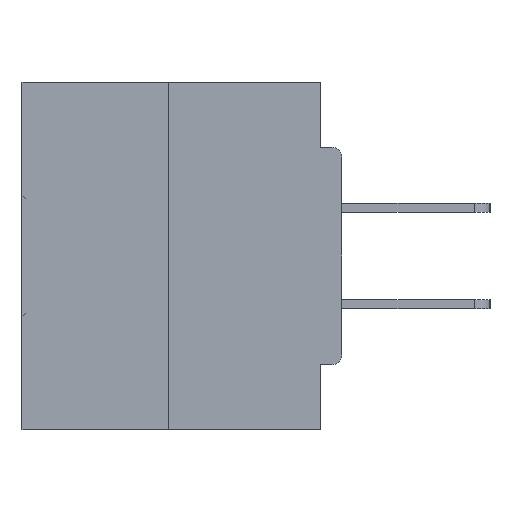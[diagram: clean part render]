
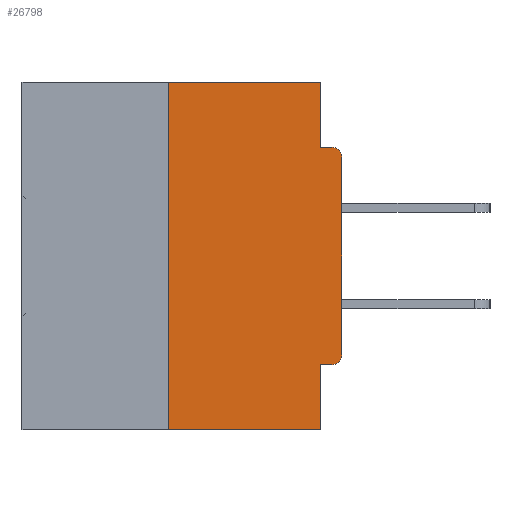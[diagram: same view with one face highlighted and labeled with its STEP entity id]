
A CAD part, left-side view. The second image highlights one B-rep face of the part: STEP entity #26798.
In plain terms, the highlighted planar face has unit normal (-1, 0, 0).
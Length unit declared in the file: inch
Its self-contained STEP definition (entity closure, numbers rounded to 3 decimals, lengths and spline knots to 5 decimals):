
#887 = LINE ( 'NONE', #7431, #6098 ) ;
#1137 = VERTEX_POINT ( 'NONE', #24487 ) ;
#1138 = ORIENTED_EDGE ( 'NONE', *, *, #22868, .F. ) ;
#1396 = DIRECTION ( 'NONE',  ( 0., 0., -1. ) ) ;
#2634 = AXIS2_PLACEMENT_3D ( 'NONE', #39475, #12281, #22226 ) ;
#2792 = ORIENTED_EDGE ( 'NONE', *, *, #13801, .T. ) ;
#3050 = ORIENTED_EDGE ( 'NONE', *, *, #20213, .F. ) ;
#3106 = CARTESIAN_POINT ( 'NONE',  ( 0., 0., -0.4065 ) ) ;
#3130 = VERTEX_POINT ( 'NONE', #12246 ) ;
#3307 = VERTEX_POINT ( 'NONE', #12253 ) ;
#3543 = EDGE_CURVE ( 'NONE', #22917, #3307, #18586, .T. ) ;
#3887 = AXIS2_PLACEMENT_3D ( 'NONE', #36619, #22894, #29551 ) ;
#4044 = VERTEX_POINT ( 'NONE', #23950 ) ;
#4377 = VERTEX_POINT ( 'NONE', #38327 ) ;
#4895 = VERTEX_POINT ( 'NONE', #5065 ) ;
#5065 = CARTESIAN_POINT ( 'NONE',  ( 0., 0., -0.3915 ) ) ;
#5417 = DIRECTION ( 'NONE',  ( 1., 0., 0. ) ) ;
#6098 = VECTOR ( 'NONE', #27663, 39.37008 ) ;
#7431 = CARTESIAN_POINT ( 'NONE',  ( 0., 0.031, 0. ) ) ;
#7897 = CARTESIAN_POINT ( 'NONE',  ( 0., 0.031, -0.5 ) ) ;
#8115 = VECTOR ( 'NONE', #10540, 39.37008 ) ;
#9086 = VERTEX_POINT ( 'NONE', #32831 ) ;
#9930 = DIRECTION ( 'NONE',  ( 0., 1., 0. ) ) ;
#9989 = EDGE_CURVE ( 'NONE', #4895, #4377, #43073, .T. ) ;
#10431 = CARTESIAN_POINT ( 'NONE',  ( 0., 0.25, 0. ) ) ;
#10540 = DIRECTION ( 'NONE',  ( 0., 0., 1. ) ) ;
#10951 = LINE ( 'NONE', #12282, #24762 ) ;
#12246 = CARTESIAN_POINT ( 'NONE',  ( 0., 0.015, -0.0935 ) ) ;
#12253 = CARTESIAN_POINT ( 'NONE',  ( 0., 0.031, -0.4065 ) ) ;
#12281 = DIRECTION ( 'NONE',  ( -1., 0., 0. ) ) ;
#12282 = CARTESIAN_POINT ( 'NONE',  ( 0., 0.46, -0.5 ) ) ;
#13551 = CARTESIAN_POINT ( 'NONE',  ( 0., 0., -0.0935 ) ) ;
#13801 = EDGE_CURVE ( 'NONE', #4044, #25861, #10951, .T. ) ;
#14295 = CARTESIAN_POINT ( 'NONE',  ( 0., 0., 0. ) ) ;
#14833 = FACE_OUTER_BOUND ( 'NONE', #15246, .T. ) ;
#15246 = EDGE_LOOP ( 'NONE', ( #38923, #3050, #2792, #34769, #36209, #39781, #43859, #40238, #1138, #22539 ) ) ;
#15605 = LINE ( 'NONE', #26620, #20967 ) ;
#17031 = EDGE_CURVE ( 'NONE', #3307, #25861, #29061, .T. ) ;
#17248 = LINE ( 'NONE', #13551, #43148 ) ;
#18035 = EDGE_CURVE ( 'NONE', #22917, #4895, #23677, .T. ) ;
#18586 = LINE ( 'NONE', #3106, #29183 ) ;
#20213 = EDGE_CURVE ( 'NONE', #4044, #42009, #39840, .T. ) ;
#20967 = VECTOR ( 'NONE', #30167, 39.37008 ) ;
#22226 = DIRECTION ( 'NONE',  ( 0., 0., -1. ) ) ;
#22364 = CARTESIAN_POINT ( 'NONE',  ( 0., 0.015, -0.4065 ) ) ;
#22539 = ORIENTED_EDGE ( 'NONE', *, *, #40933, .F. ) ;
#22868 = EDGE_CURVE ( 'NONE', #9086, #3130, #17248, .T. ) ;
#22894 = DIRECTION ( 'NONE',  ( -1., 0., 0. ) ) ;
#22917 = VERTEX_POINT ( 'NONE', #22364 ) ;
#23013 = EDGE_CURVE ( 'NONE', #42009, #1137, #15605, .T. ) ;
#23677 = CIRCLE ( 'NONE', #2634, 0.015 ) ;
#23950 = CARTESIAN_POINT ( 'NONE',  ( 0., 0.25, -0.5 ) ) ;
#24487 = CARTESIAN_POINT ( 'NONE',  ( 0., 0.031, 0. ) ) ;
#24762 = VECTOR ( 'NONE', #29306, 39.37008 ) ;
#25861 = VERTEX_POINT ( 'NONE', #43843 ) ;
#26620 = CARTESIAN_POINT ( 'NONE',  ( 0., 0.46, 0. ) ) ;
#26798 = ADVANCED_FACE ( 'NONE', ( #14833 ), #32436, .F. ) ;
#27365 = AXIS2_PLACEMENT_3D ( 'NONE', #39230, #5417, #29202 ) ;
#27663 = DIRECTION ( 'NONE',  ( 0., 0., -1. ) ) ;
#28241 = CARTESIAN_POINT ( 'NONE',  ( 0., 0.25, 0. ) ) ;
#29061 = LINE ( 'NONE', #7897, #37546 ) ;
#29183 = VECTOR ( 'NONE', #9930, 39.37008 ) ;
#29202 = DIRECTION ( 'NONE',  ( 0., 0., -1. ) ) ;
#29306 = DIRECTION ( 'NONE',  ( 0., -1., 0. ) ) ;
#29551 = DIRECTION ( 'NONE',  ( 0., 0., -1. ) ) ;
#29802 = VECTOR ( 'NONE', #37323, 39.37008 ) ;
#30167 = DIRECTION ( 'NONE',  ( 0., -1., 0. ) ) ;
#32436 = PLANE ( 'NONE',  #27365 ) ;
#32831 = CARTESIAN_POINT ( 'NONE',  ( 0., 0.031, -0.0935 ) ) ;
#34769 = ORIENTED_EDGE ( 'NONE', *, *, #17031, .F. ) ;
#36209 = ORIENTED_EDGE ( 'NONE', *, *, #3543, .F. ) ;
#36280 = CIRCLE ( 'NONE', #3887, 0.015 ) ;
#36619 = CARTESIAN_POINT ( 'NONE',  ( 0., 0.015, -0.1085 ) ) ;
#37323 = DIRECTION ( 'NONE',  ( 0., 0., 1. ) ) ;
#37546 = VECTOR ( 'NONE', #1396, 39.37008 ) ;
#38243 = DIRECTION ( 'NONE',  ( 0., -1., 0. ) ) ;
#38327 = CARTESIAN_POINT ( 'NONE',  ( 0., 0., -0.1085 ) ) ;
#38923 = ORIENTED_EDGE ( 'NONE', *, *, #23013, .F. ) ;
#39230 = CARTESIAN_POINT ( 'NONE',  ( 0., 0.46, 0. ) ) ;
#39475 = CARTESIAN_POINT ( 'NONE',  ( 0., 0.015, -0.3915 ) ) ;
#39781 = ORIENTED_EDGE ( 'NONE', *, *, #18035, .T. ) ;
#39840 = LINE ( 'NONE', #10431, #29802 ) ;
#40238 = ORIENTED_EDGE ( 'NONE', *, *, #41717, .T. ) ;
#40933 = EDGE_CURVE ( 'NONE', #1137, #9086, #887, .T. ) ;
#41717 = EDGE_CURVE ( 'NONE', #4377, #3130, #36280, .T. ) ;
#42009 = VERTEX_POINT ( 'NONE', #28241 ) ;
#43073 = LINE ( 'NONE', #14295, #8115 ) ;
#43148 = VECTOR ( 'NONE', #38243, 39.37008 ) ;
#43843 = CARTESIAN_POINT ( 'NONE',  ( 0., 0.031, -0.5 ) ) ;
#43859 = ORIENTED_EDGE ( 'NONE', *, *, #9989, .T. ) ;
